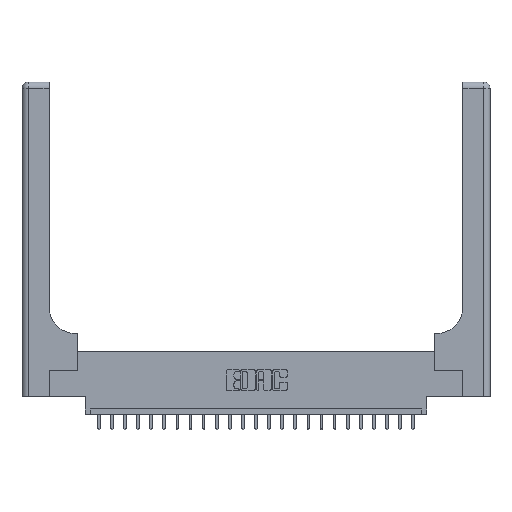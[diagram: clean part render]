
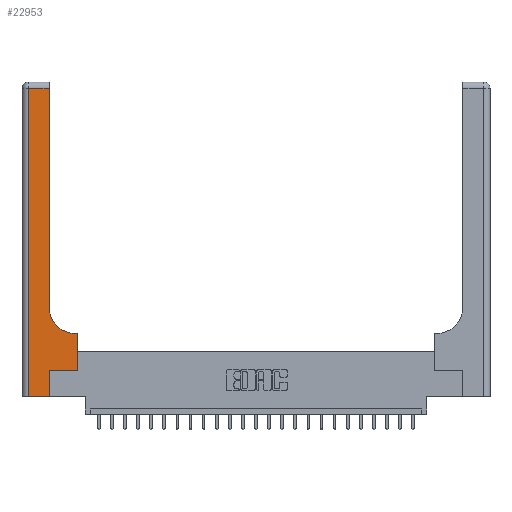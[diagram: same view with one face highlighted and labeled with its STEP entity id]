
A CAD part, top view. The second image highlights one B-rep face of the part: STEP entity #22953.
In plain terms, the highlighted planar face has unit normal (0, 0, 1).
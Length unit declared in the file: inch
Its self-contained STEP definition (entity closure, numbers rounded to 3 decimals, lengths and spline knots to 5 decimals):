
#300 = VERTEX_POINT ( 'NONE', #7423 ) ;
#344 = EDGE_LOOP ( 'NONE', ( #22589, #5283, #16432, #757, #22812, #22415, #7975, #4324, #10412 ) ) ;
#350 = EDGE_CURVE ( 'NONE', #5920, #2994, #11615, .T. ) ;
#436 = VECTOR ( 'NONE', #2318, 39.37008 ) ;
#665 = DIRECTION ( 'NONE',  ( 0., 0., -1. ) ) ;
#757 = ORIENTED_EDGE ( 'NONE', *, *, #21568, .T. ) ;
#856 = VECTOR ( 'NONE', #7177, 39.37008 ) ;
#1168 = VECTOR ( 'NONE', #2847, 39.37008 ) ;
#1256 = VERTEX_POINT ( 'NONE', #17942 ) ;
#1588 = DIRECTION ( 'NONE',  ( 0., 1., 0. ) ) ;
#1653 = LINE ( 'NONE', #14325, #15050 ) ;
#1921 = PLANE ( 'NONE',  #10487 ) ;
#2176 = CIRCLE ( 'NONE', #15929, 0.25 ) ;
#2318 = DIRECTION ( 'NONE',  ( 0., 1., 0. ) ) ;
#2446 = DIRECTION ( 'NONE',  ( 1., 0., 0. ) ) ;
#2847 = DIRECTION ( 'NONE',  ( -1., 0., 0. ) ) ;
#2994 = VERTEX_POINT ( 'NONE', #17810 ) ;
#3317 = VECTOR ( 'NONE', #1588, 39.37008 ) ;
#3478 = DIRECTION ( 'NONE',  ( 0., 0., -1. ) ) ;
#3785 = VERTEX_POINT ( 'NONE', #20972 ) ;
#4150 = LINE ( 'NONE', #8212, #11911 ) ;
#4324 = ORIENTED_EDGE ( 'NONE', *, *, #18884, .T. ) ;
#4411 = EDGE_CURVE ( 'NONE', #2994, #8978, #20298, .T. ) ;
#5029 = VECTOR ( 'NONE', #12737, 39.37008 ) ;
#5203 = LINE ( 'NONE', #5438, #5029 ) ;
#5283 = ORIENTED_EDGE ( 'NONE', *, *, #8759, .T. ) ;
#5438 = CARTESIAN_POINT ( 'NONE',  ( 0.06, 3., 0.37 ) ) ;
#5859 = VERTEX_POINT ( 'NONE', #17452 ) ;
#5920 = VERTEX_POINT ( 'NONE', #22061 ) ;
#6237 = DIRECTION ( 'NONE',  ( 0., 1., 0. ) ) ;
#7177 = DIRECTION ( 'NONE',  ( 1., 0., 0. ) ) ;
#7423 = CARTESIAN_POINT ( 'NONE',  ( 0.06, 0., 0.37 ) ) ;
#7652 = FACE_OUTER_BOUND ( 'NONE', #344, .T. ) ;
#7975 = ORIENTED_EDGE ( 'NONE', *, *, #12430, .T. ) ;
#8212 = CARTESIAN_POINT ( 'NONE',  ( 0.26, 0.6, 0.37 ) ) ;
#8759 = EDGE_CURVE ( 'NONE', #1256, #10982, #11812, .T. ) ;
#8978 = VERTEX_POINT ( 'NONE', #12400 ) ;
#8992 = LINE ( 'NONE', #10552, #3317 ) ;
#10412 = ORIENTED_EDGE ( 'NONE', *, *, #12223, .T. ) ;
#10487 = AXIS2_PLACEMENT_3D ( 'NONE', #14597, #3478, #18293 ) ;
#10552 = CARTESIAN_POINT ( 'NONE',  ( 0.528, 0.25, 0.37 ) ) ;
#10982 = VERTEX_POINT ( 'NONE', #14258 ) ;
#11541 = CARTESIAN_POINT ( 'NONE',  ( 0.51, 0.85, 0.37 ) ) ;
#11615 = LINE ( 'NONE', #18649, #19680 ) ;
#11812 = LINE ( 'NONE', #13488, #1168 ) ;
#11911 = VECTOR ( 'NONE', #13469, 39.37008 ) ;
#12223 = EDGE_CURVE ( 'NONE', #21301, #5859, #2176, .T. ) ;
#12400 = CARTESIAN_POINT ( 'NONE',  ( 0.528, 0.25, 0.37 ) ) ;
#12430 = EDGE_CURVE ( 'NONE', #8978, #3785, #8992, .T. ) ;
#12737 = DIRECTION ( 'NONE',  ( 0., -1., 0. ) ) ;
#13073 = CARTESIAN_POINT ( 'NONE',  ( 0.51, 0.6, 0.37 ) ) ;
#13196 = LINE ( 'NONE', #14632, #436 ) ;
#13469 = DIRECTION ( 'NONE',  ( -1., 0., 0. ) ) ;
#13488 = CARTESIAN_POINT ( 'NONE',  ( 0., 2.94, 0.37 ) ) ;
#14258 = CARTESIAN_POINT ( 'NONE',  ( 0.06, 2.94, 0.37 ) ) ;
#14325 = CARTESIAN_POINT ( 'NONE',  ( 0., 0., 0.37 ) ) ;
#14597 = CARTESIAN_POINT ( 'NONE',  ( 0., 3., 0.37 ) ) ;
#14632 = CARTESIAN_POINT ( 'NONE',  ( 0.26, 3., 0.37 ) ) ;
#15050 = VECTOR ( 'NONE', #21828, 39.37008 ) ;
#15929 = AXIS2_PLACEMENT_3D ( 'NONE', #11541, #665, #2446 ) ;
#16149 = CARTESIAN_POINT ( 'NONE',  ( 0.265, 0.25, 0.37 ) ) ;
#16303 = EDGE_CURVE ( 'NONE', #5859, #1256, #13196, .T. ) ;
#16432 = ORIENTED_EDGE ( 'NONE', *, *, #19242, .T. ) ;
#17452 = CARTESIAN_POINT ( 'NONE',  ( 0.26, 0.85, 0.37 ) ) ;
#17810 = CARTESIAN_POINT ( 'NONE',  ( 0.265, 0.25, 0.37 ) ) ;
#17942 = CARTESIAN_POINT ( 'NONE',  ( 0.26, 2.94, 0.37 ) ) ;
#18293 = DIRECTION ( 'NONE',  ( -1., 0., 0. ) ) ;
#18649 = CARTESIAN_POINT ( 'NONE',  ( 0.265, 0., 0.37 ) ) ;
#18884 = EDGE_CURVE ( 'NONE', #3785, #21301, #4150, .T. ) ;
#19242 = EDGE_CURVE ( 'NONE', #10982, #300, #5203, .T. ) ;
#19680 = VECTOR ( 'NONE', #6237, 39.37008 ) ;
#20298 = LINE ( 'NONE', #16149, #856 ) ;
#20972 = CARTESIAN_POINT ( 'NONE',  ( 0.528, 0.6, 0.37 ) ) ;
#21301 = VERTEX_POINT ( 'NONE', #13073 ) ;
#21568 = EDGE_CURVE ( 'NONE', #300, #5920, #1653, .T. ) ;
#21828 = DIRECTION ( 'NONE',  ( 1., 0., 0. ) ) ;
#22061 = CARTESIAN_POINT ( 'NONE',  ( 0.265, 0., 0.37 ) ) ;
#22415 = ORIENTED_EDGE ( 'NONE', *, *, #4411, .T. ) ;
#22589 = ORIENTED_EDGE ( 'NONE', *, *, #16303, .T. ) ;
#22812 = ORIENTED_EDGE ( 'NONE', *, *, #350, .T. ) ;
#22953 = ADVANCED_FACE ( 'NONE', ( #7652 ), #1921, .F. ) ;
